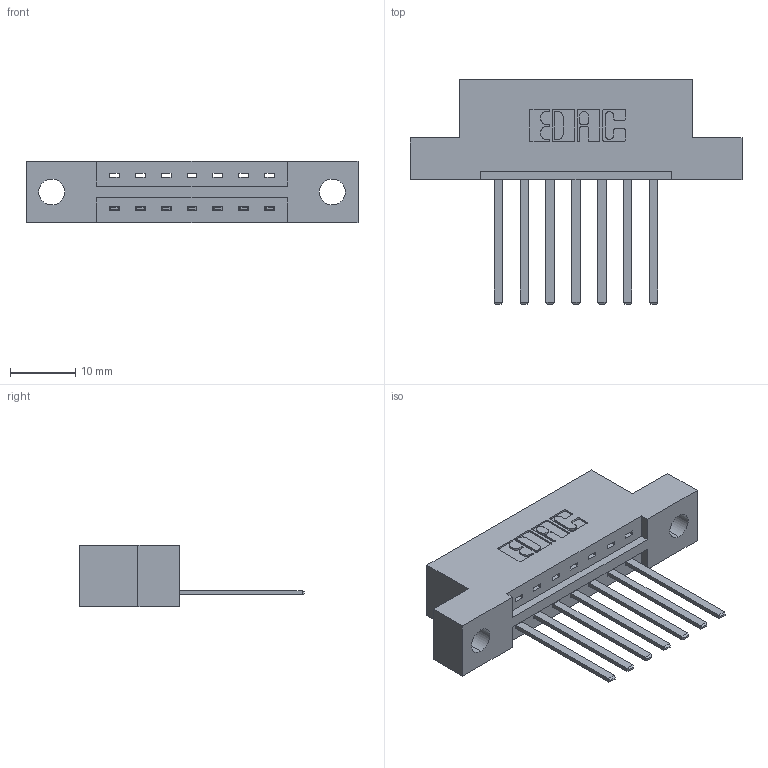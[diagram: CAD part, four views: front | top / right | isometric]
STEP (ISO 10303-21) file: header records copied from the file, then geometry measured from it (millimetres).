
FILE_DESCRIPTION (( 'STEP AP203' ), '1' );
FILE_NAME ('337-007-544-104.STEP', '2018-08-03T20:26:55', ( '' ), ( '' ), 'SwSTEP 2.0', 'SolidWorks 2016', '' );
FILE_SCHEMA (( 'CONFIG_CONTROL_DESIGN' ));
Length unit declared in the file: inch
Products named in the file (3): 337 Part_Flush Mounting Lugs - 0.156 Dia-TH; 345-292-001_345-293-144; 337-007-544-104
Assembly tree (8 placements, depth 2):
  337-007-544-104
    337 Part_Flush Mounting Lugs - 0.156 Dia-TH
    345-292-001_345-293-144  x7
Bounding box: 50.75 x 34.3 x 9.4 mm (x, y, z)
Volume: 4829.8 mm3; surface area: 4858.6 mm2
Topology: 8 solids, 8 shells, 506 faces, 1501 edges, 990 vertices
Faces by surface type: plane 364, cylinder 142
Entity records: 9549 total; most frequent: CARTESIAN_POINT 1667, ORIENTED_EDGE 1610, DIRECTION 1471, EDGE_CURVE 805, LINE 681, VECTOR 681, VERTEX_POINT 534, AXIS2_PLACEMENT_3D 395
